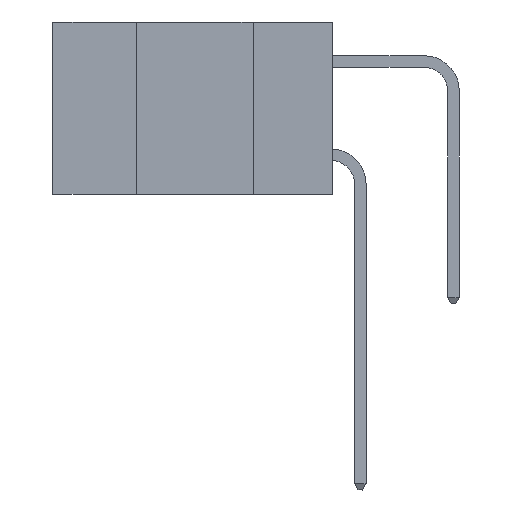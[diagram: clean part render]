
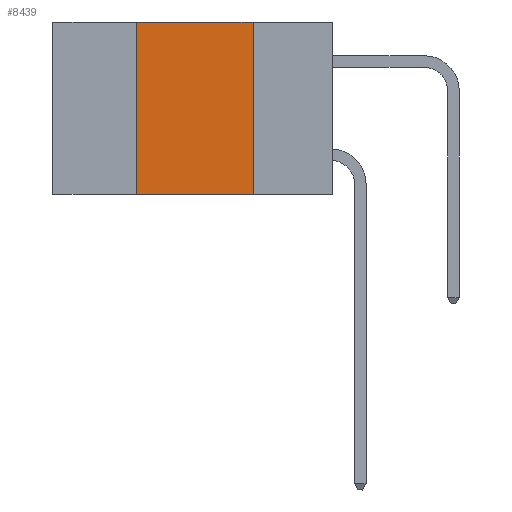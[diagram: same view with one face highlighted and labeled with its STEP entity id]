
A CAD part, left-side view. The second image highlights one B-rep face of the part: STEP entity #8439.
In plain terms, the highlighted planar face has unit normal (-1, 0, 0).
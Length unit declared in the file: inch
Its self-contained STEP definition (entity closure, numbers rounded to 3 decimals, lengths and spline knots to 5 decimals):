
#56 = ORIENTED_EDGE ( 'NONE', *, *, #2505, .F. ) ;
#566 = CARTESIAN_POINT ( 'NONE',  ( 0., 0.17, 0. ) ) ;
#610 = VERTEX_POINT ( 'NONE', #28031 ) ;
#1727 = DIRECTION ( 'NONE',  ( 0., -1., 0. ) ) ;
#2018 = FACE_OUTER_BOUND ( 'NONE', #28220, .T. ) ;
#2505 = EDGE_CURVE ( 'NONE', #16687, #11531, #23574, .T. ) ;
#3844 = PLANE ( 'NONE',  #17785 ) ;
#3921 = LINE ( 'NONE', #9274, #15892 ) ;
#7331 = EDGE_CURVE ( 'NONE', #610, #17584, #27079, .T. ) ;
#8089 = CARTESIAN_POINT ( 'NONE',  ( 0., 0.42, 0. ) ) ;
#8439 = ADVANCED_FACE ( 'NONE', ( #2018 ), #3844, .F. ) ;
#8664 = DIRECTION ( 'NONE',  ( 0., 0., -1. ) ) ;
#9274 = CARTESIAN_POINT ( 'NONE',  ( 0., 0.6, -0.37 ) ) ;
#10693 = VECTOR ( 'NONE', #15452, 39.37008 ) ;
#11265 = CARTESIAN_POINT ( 'NONE',  ( 0., 0.6, 0. ) ) ;
#11531 = VERTEX_POINT ( 'NONE', #27583 ) ;
#15452 = DIRECTION ( 'NONE',  ( 0., 0., -1. ) ) ;
#15892 = VECTOR ( 'NONE', #28655, 39.37008 ) ;
#16687 = VERTEX_POINT ( 'NONE', #27992 ) ;
#17584 = VERTEX_POINT ( 'NONE', #19238 ) ;
#17672 = VECTOR ( 'NONE', #1727, 39.37008 ) ;
#17785 = AXIS2_PLACEMENT_3D ( 'NONE', #20705, #23131, #8664 ) ;
#18639 = EDGE_CURVE ( 'NONE', #17584, #16687, #24175, .T. ) ;
#19238 = CARTESIAN_POINT ( 'NONE',  ( 0., 0.42, 0. ) ) ;
#20583 = VECTOR ( 'NONE', #21822, 39.37008 ) ;
#20705 = CARTESIAN_POINT ( 'NONE',  ( 0., 0.6, 0. ) ) ;
#20886 = EDGE_CURVE ( 'NONE', #610, #11531, #3921, .T. ) ;
#21214 = ORIENTED_EDGE ( 'NONE', *, *, #20886, .T. ) ;
#21822 = DIRECTION ( 'NONE',  ( 0., 0., 1. ) ) ;
#23131 = DIRECTION ( 'NONE',  ( 1., 0., 0. ) ) ;
#23574 = LINE ( 'NONE', #566, #10693 ) ;
#24175 = LINE ( 'NONE', #11265, #17672 ) ;
#25365 = ORIENTED_EDGE ( 'NONE', *, *, #18639, .F. ) ;
#25757 = ORIENTED_EDGE ( 'NONE', *, *, #7331, .F. ) ;
#27079 = LINE ( 'NONE', #8089, #20583 ) ;
#27583 = CARTESIAN_POINT ( 'NONE',  ( 0., 0.17, -0.37 ) ) ;
#27992 = CARTESIAN_POINT ( 'NONE',  ( 0., 0.17, 0. ) ) ;
#28031 = CARTESIAN_POINT ( 'NONE',  ( 0., 0.42, -0.37 ) ) ;
#28220 = EDGE_LOOP ( 'NONE', ( #56, #25365, #25757, #21214 ) ) ;
#28655 = DIRECTION ( 'NONE',  ( 0., -1., 0. ) ) ;
